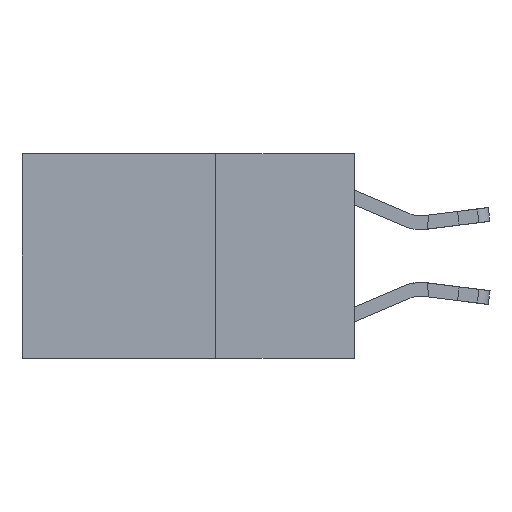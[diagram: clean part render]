
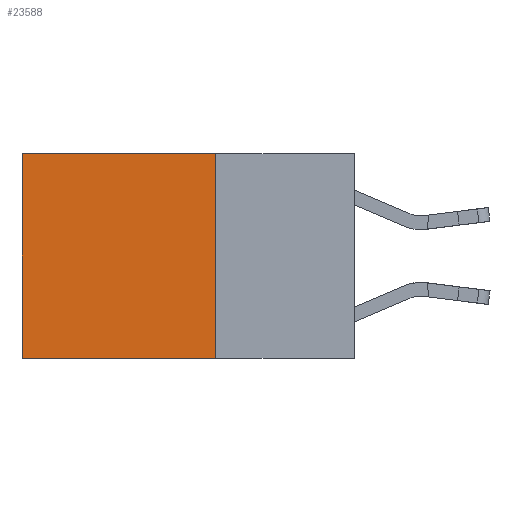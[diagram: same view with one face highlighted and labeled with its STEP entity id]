
A CAD part, left-side view. The second image highlights one B-rep face of the part: STEP entity #23588.
In plain terms, the highlighted planar face has unit normal (-1, 0, 0).
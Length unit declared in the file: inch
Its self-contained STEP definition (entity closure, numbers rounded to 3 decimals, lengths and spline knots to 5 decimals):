
#682 = EDGE_CURVE ( 'NONE', #24950, #11319, #19254, .T. ) ;
#923 = CARTESIAN_POINT ( 'NONE',  ( 0.2625, 0.6, 0. ) ) ;
#1496 = VECTOR ( 'NONE', #2966, 39.37008 ) ;
#2344 = ORIENTED_EDGE ( 'NONE', *, *, #682, .T. ) ;
#2966 = DIRECTION ( 'NONE',  ( 0., 0., -1. ) ) ;
#4118 = CARTESIAN_POINT ( 'NONE',  ( 0.2625, 0.25, 0. ) ) ;
#4144 = CARTESIAN_POINT ( 'NONE',  ( 0.2625, 0.25, 0. ) ) ;
#4421 = FACE_OUTER_BOUND ( 'NONE', #9295, .T. ) ;
#4422 = EDGE_CURVE ( 'NONE', #19101, #12426, #16299, .T. ) ;
#4782 = DIRECTION ( 'NONE',  ( 0., 1., 0. ) ) ;
#7259 = CARTESIAN_POINT ( 'NONE',  ( 0.2625, 0.25, -0.37 ) ) ;
#8094 = DIRECTION ( 'NONE',  ( 0., 0., -1. ) ) ;
#9295 = EDGE_LOOP ( 'NONE', ( #2344, #24488, #9745, #22261 ) ) ;
#9383 = EDGE_CURVE ( 'NONE', #12426, #11319, #25131, .T. ) ;
#9745 = ORIENTED_EDGE ( 'NONE', *, *, #4422, .F. ) ;
#11319 = VERTEX_POINT ( 'NONE', #12066 ) ;
#11837 = DIRECTION ( 'NONE',  ( 0., 1., 0. ) ) ;
#12066 = CARTESIAN_POINT ( 'NONE',  ( 0.2625, 0.6, -0.37 ) ) ;
#12423 = VECTOR ( 'NONE', #11837, 39.37008 ) ;
#12426 = VERTEX_POINT ( 'NONE', #7259 ) ;
#12759 = CARTESIAN_POINT ( 'NONE',  ( 0.2625, 0.6, 0. ) ) ;
#15275 = VECTOR ( 'NONE', #4782, 39.37008 ) ;
#16299 = LINE ( 'NONE', #26557, #23183 ) ;
#16635 = CARTESIAN_POINT ( 'NONE',  ( 0.2625, 0.25, -0.37 ) ) ;
#16674 = DIRECTION ( 'NONE',  ( 1., 0., 0. ) ) ;
#16862 = EDGE_CURVE ( 'NONE', #19101, #24950, #21968, .T. ) ;
#19101 = VERTEX_POINT ( 'NONE', #4118 ) ;
#19254 = LINE ( 'NONE', #923, #1496 ) ;
#20849 = PLANE ( 'NONE',  #21077 ) ;
#20984 = DIRECTION ( 'NONE',  ( 0., 0., -1. ) ) ;
#21077 = AXIS2_PLACEMENT_3D ( 'NONE', #4144, #16674, #20984 ) ;
#21968 = LINE ( 'NONE', #26020, #12423 ) ;
#22261 = ORIENTED_EDGE ( 'NONE', *, *, #16862, .T. ) ;
#23183 = VECTOR ( 'NONE', #8094, 39.37008 ) ;
#23588 = ADVANCED_FACE ( 'NONE', ( #4421 ), #20849, .F. ) ;
#24488 = ORIENTED_EDGE ( 'NONE', *, *, #9383, .F. ) ;
#24950 = VERTEX_POINT ( 'NONE', #12759 ) ;
#25131 = LINE ( 'NONE', #16635, #15275 ) ;
#26020 = CARTESIAN_POINT ( 'NONE',  ( 0.2625, 0.25, 0. ) ) ;
#26557 = CARTESIAN_POINT ( 'NONE',  ( 0.2625, 0.25, 0. ) ) ;
